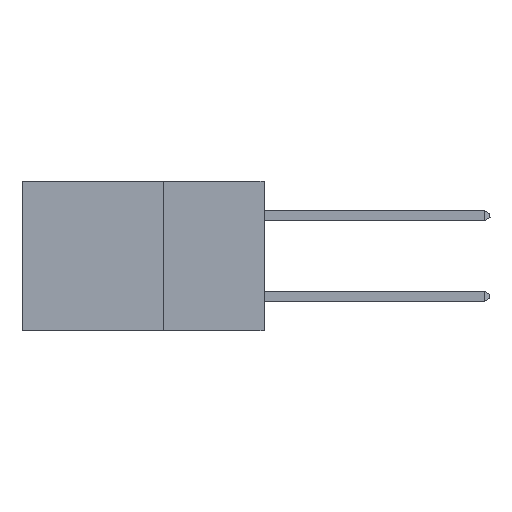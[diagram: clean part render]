
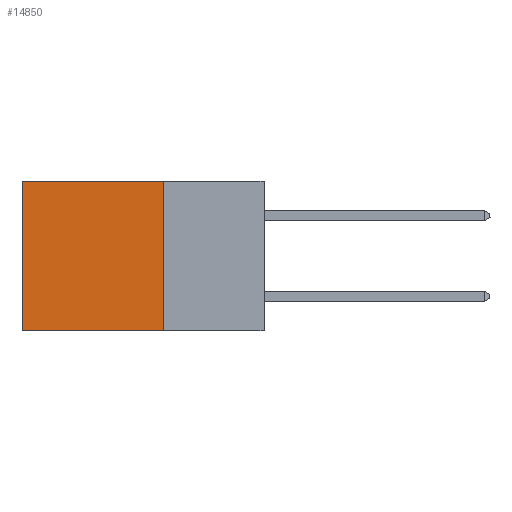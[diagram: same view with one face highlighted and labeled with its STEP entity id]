
A CAD part, left-side view. The second image highlights one B-rep face of the part: STEP entity #14850.
In plain terms, the highlighted planar face has unit normal (-1, 0, 0).
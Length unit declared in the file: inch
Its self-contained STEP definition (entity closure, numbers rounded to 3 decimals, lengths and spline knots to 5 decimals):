
#513 = ORIENTED_EDGE ( 'NONE', *, *, #12014, .F. ) ;
#637 = DIRECTION ( 'NONE',  ( 0., 0., -1. ) ) ;
#1167 = CARTESIAN_POINT ( 'NONE',  ( 0.298, 0.25, -0.37 ) ) ;
#1180 = DIRECTION ( 'NONE',  ( 0., 1., 0. ) ) ;
#1209 = CARTESIAN_POINT ( 'NONE',  ( 0.298, 0.25, 0. ) ) ;
#1578 = EDGE_CURVE ( 'NONE', #15580, #8123, #1814, .T. ) ;
#1814 = LINE ( 'NONE', #14313, #8458 ) ;
#2565 = CARTESIAN_POINT ( 'NONE',  ( 0.298, 0.25, 0. ) ) ;
#2995 = ORIENTED_EDGE ( 'NONE', *, *, #10497, .F. ) ;
#5012 = EDGE_CURVE ( 'NONE', #8123, #7706, #5178, .T. ) ;
#5178 = LINE ( 'NONE', #7470, #14846 ) ;
#5947 = VECTOR ( 'NONE', #1180, 39.37008 ) ;
#6792 = LINE ( 'NONE', #16791, #5947 ) ;
#7470 = CARTESIAN_POINT ( 'NONE',  ( 0.298, 0.6, 0. ) ) ;
#7706 = VERTEX_POINT ( 'NONE', #8229 ) ;
#8045 = EDGE_LOOP ( 'NONE', ( #9329, #2995, #513, #15761 ) ) ;
#8123 = VERTEX_POINT ( 'NONE', #14869 ) ;
#8229 = CARTESIAN_POINT ( 'NONE',  ( 0.298, 0.6, -0.37 ) ) ;
#8379 = VECTOR ( 'NONE', #9030, 39.37008 ) ;
#8458 = VECTOR ( 'NONE', #10609, 39.37008 ) ;
#8563 = VERTEX_POINT ( 'NONE', #1167 ) ;
#9030 = DIRECTION ( 'NONE',  ( 0., 0., -1. ) ) ;
#9329 = ORIENTED_EDGE ( 'NONE', *, *, #5012, .T. ) ;
#9634 = FACE_OUTER_BOUND ( 'NONE', #8045, .T. ) ;
#9800 = DIRECTION ( 'NONE',  ( 0., 0., -1. ) ) ;
#10486 = LINE ( 'NONE', #2565, #8379 ) ;
#10497 = EDGE_CURVE ( 'NONE', #8563, #7706, #6792, .T. ) ;
#10609 = DIRECTION ( 'NONE',  ( 0., 1., 0. ) ) ;
#11049 = AXIS2_PLACEMENT_3D ( 'NONE', #13835, #12577, #9800 ) ;
#12014 = EDGE_CURVE ( 'NONE', #15580, #8563, #10486, .T. ) ;
#12577 = DIRECTION ( 'NONE',  ( 1., 0., 0. ) ) ;
#13835 = CARTESIAN_POINT ( 'NONE',  ( 0.298, 0.25, 0. ) ) ;
#14313 = CARTESIAN_POINT ( 'NONE',  ( 0.298, 0.25, 0. ) ) ;
#14846 = VECTOR ( 'NONE', #637, 39.37008 ) ;
#14850 = ADVANCED_FACE ( 'NONE', ( #9634 ), #14997, .F. ) ;
#14869 = CARTESIAN_POINT ( 'NONE',  ( 0.298, 0.6, 0. ) ) ;
#14997 = PLANE ( 'NONE',  #11049 ) ;
#15580 = VERTEX_POINT ( 'NONE', #1209 ) ;
#15761 = ORIENTED_EDGE ( 'NONE', *, *, #1578, .T. ) ;
#16791 = CARTESIAN_POINT ( 'NONE',  ( 0.298, 0.25, -0.37 ) ) ;
